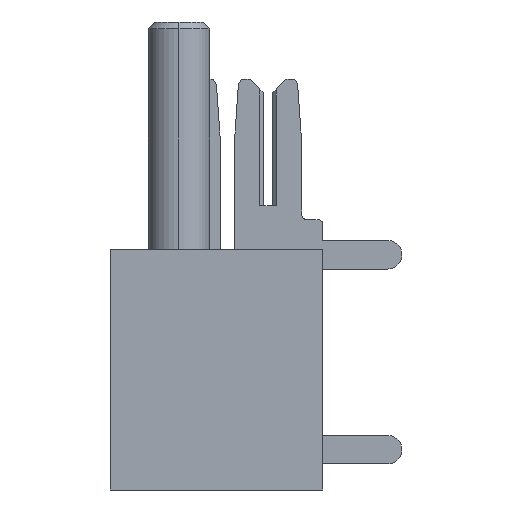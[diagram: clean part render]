
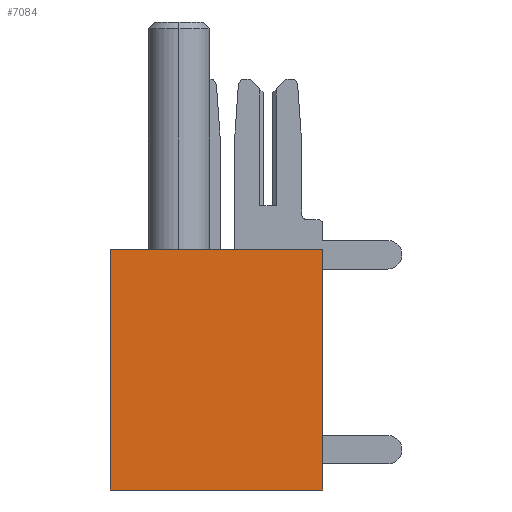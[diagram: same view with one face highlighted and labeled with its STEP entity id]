
A CAD part, left-side view. The second image highlights one B-rep face of the part: STEP entity #7084.
In plain terms, the highlighted planar face has unit normal (-1, 0, 0).
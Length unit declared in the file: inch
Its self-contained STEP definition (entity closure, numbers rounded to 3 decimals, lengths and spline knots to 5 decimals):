
#20 = CARTESIAN_POINT ( 'NONE',  ( 0., 0., 0. ) ) ;
#46 = DIRECTION ( 'NONE',  ( 0., 0., 1. ) ) ;
#113 = CARTESIAN_POINT ( 'NONE',  ( 0., 0.327, -0.37 ) ) ;
#337 = VECTOR ( 'NONE', #2994, 39.37008 ) ;
#579 = VERTEX_POINT ( 'NONE', #787 ) ;
#787 = CARTESIAN_POINT ( 'NONE',  ( 0., 0., 0. ) ) ;
#867 = EDGE_CURVE ( 'NONE', #2821, #4665, #8745, .T. ) ;
#1123 = CARTESIAN_POINT ( 'NONE',  ( 0., 0., -0.37 ) ) ;
#1184 = DIRECTION ( 'NONE',  ( -1., 0., 0. ) ) ;
#1279 = DIRECTION ( 'NONE',  ( 0., 0., 1. ) ) ;
#1771 = AXIS2_PLACEMENT_3D ( 'NONE', #5595, #1184, #1279 ) ;
#2202 = ORIENTED_EDGE ( 'NONE', *, *, #3085, .T. ) ;
#2436 = CARTESIAN_POINT ( 'NONE',  ( 0., 0., -0.37 ) ) ;
#2645 = ORIENTED_EDGE ( 'NONE', *, *, #6676, .F. ) ;
#2821 = VERTEX_POINT ( 'NONE', #5476 ) ;
#2994 = DIRECTION ( 'NONE',  ( 0., -1., 0. ) ) ;
#3085 = EDGE_CURVE ( 'NONE', #4665, #579, #6460, .T. ) ;
#3121 = DIRECTION ( 'NONE',  ( 0., 0., 1. ) ) ;
#3588 = DIRECTION ( 'NONE',  ( 0., -1., 0. ) ) ;
#4596 = EDGE_CURVE ( 'NONE', #5294, #579, #6709, .T. ) ;
#4665 = VERTEX_POINT ( 'NONE', #2436 ) ;
#5024 = PLANE ( 'NONE',  #1771 ) ;
#5101 = ORIENTED_EDGE ( 'NONE', *, *, #4596, .F. ) ;
#5134 = VECTOR ( 'NONE', #3588, 39.37008 ) ;
#5294 = VERTEX_POINT ( 'NONE', #5325 ) ;
#5325 = CARTESIAN_POINT ( 'NONE',  ( 0., 0.327, 0. ) ) ;
#5476 = CARTESIAN_POINT ( 'NONE',  ( 0., 0.327, -0.37 ) ) ;
#5595 = CARTESIAN_POINT ( 'NONE',  ( 0., 0., -0.37 ) ) ;
#6460 = LINE ( 'NONE', #7238, #8623 ) ;
#6676 = EDGE_CURVE ( 'NONE', #2821, #5294, #9385, .T. ) ;
#6709 = LINE ( 'NONE', #20, #337 ) ;
#6713 = EDGE_LOOP ( 'NONE', ( #5101, #2645, #7803, #2202 ) ) ;
#7084 = ADVANCED_FACE ( 'NONE', ( #8334 ), #5024, .T. ) ;
#7238 = CARTESIAN_POINT ( 'NONE',  ( 0., 0., -0.37 ) ) ;
#7423 = VECTOR ( 'NONE', #46, 39.37008 ) ;
#7803 = ORIENTED_EDGE ( 'NONE', *, *, #867, .T. ) ;
#8334 = FACE_OUTER_BOUND ( 'NONE', #6713, .T. ) ;
#8623 = VECTOR ( 'NONE', #3121, 39.37008 ) ;
#8745 = LINE ( 'NONE', #1123, #5134 ) ;
#9385 = LINE ( 'NONE', #113, #7423 ) ;
